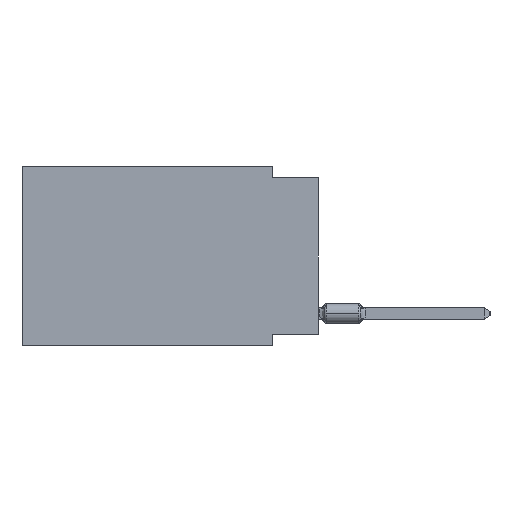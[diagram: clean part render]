
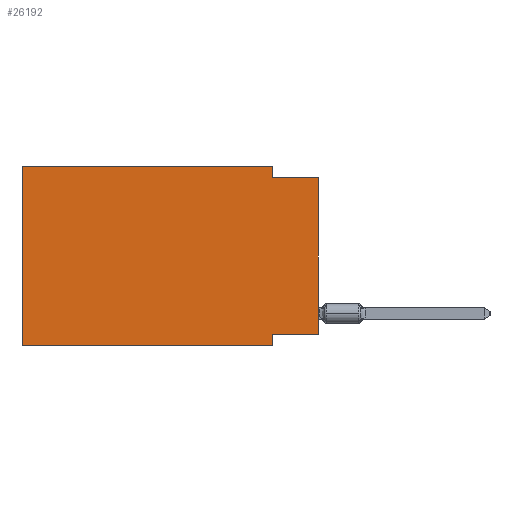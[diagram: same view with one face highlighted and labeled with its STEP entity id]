
A CAD part, left-side view. The second image highlights one B-rep face of the part: STEP entity #26192.
In plain terms, the highlighted planar face has unit normal (-1, 0, 0).
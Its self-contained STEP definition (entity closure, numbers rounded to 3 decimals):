
#17 = LINE ( 'NONE', #34394, #35979 ) ;
#1350 = EDGE_CURVE ( 'NONE', #41954, #53460, #18862, .T. ) ;
#2189 = LINE ( 'NONE', #27979, #35360 ) ;
#2396 = VERTEX_POINT ( 'NONE', #54322 ) ;
#2655 = AXIS2_PLACEMENT_3D ( 'NONE', #14996, #14698, #49918 ) ;
#2933 = CARTESIAN_POINT ( 'NONE',  ( 0., 0., -9.271 ) ) ;
#3360 = CARTESIAN_POINT ( 'NONE',  ( 0., 2.54, -9.906 ) ) ;
#4289 = CARTESIAN_POINT ( 'NONE',  ( 0., 2.54, 0. ) ) ;
#4582 = VECTOR ( 'NONE', #33559, 1000. ) ;
#6102 = PLANE ( 'NONE',  #2655 ) ;
#6469 = DIRECTION ( 'NONE',  ( 0., -1., 0. ) ) ;
#6684 = FACE_OUTER_BOUND ( 'NONE', #40012, .T. ) ;
#9177 = DIRECTION ( 'NONE',  ( 0., 0., 1. ) ) ;
#11233 = VECTOR ( 'NONE', #36967, 1000. ) ;
#11398 = DIRECTION ( 'NONE',  ( 0., 0., -1. ) ) ;
#14305 = ORIENTED_EDGE ( 'NONE', *, *, #56069, .F. ) ;
#14698 = DIRECTION ( 'NONE',  ( 1., 0., 0. ) ) ;
#14996 = CARTESIAN_POINT ( 'NONE',  ( 0., 16.383, 0. ) ) ;
#16462 = CARTESIAN_POINT ( 'NONE',  ( 0., 0., -0.635 ) ) ;
#17067 = ORIENTED_EDGE ( 'NONE', *, *, #1350, .T. ) ;
#17804 = ORIENTED_EDGE ( 'NONE', *, *, #56601, .F. ) ;
#18772 = ORIENTED_EDGE ( 'NONE', *, *, #55075, .F. ) ;
#18862 = LINE ( 'NONE', #40323, #44208 ) ;
#18875 = LINE ( 'NONE', #53771, #22609 ) ;
#19514 = LINE ( 'NONE', #46384, #11233 ) ;
#19991 = VERTEX_POINT ( 'NONE', #52858 ) ;
#20085 = EDGE_CURVE ( 'NONE', #2396, #51063, #2189, .T. ) ;
#20477 = CARTESIAN_POINT ( 'NONE',  ( 0., 0., -0.635 ) ) ;
#20501 = EDGE_CURVE ( 'NONE', #51063, #19991, #18875, .T. ) ;
#20952 = CARTESIAN_POINT ( 'NONE',  ( 0., 2.54, -9.906 ) ) ;
#22609 = VECTOR ( 'NONE', #27759, 1000. ) ;
#24961 = ORIENTED_EDGE ( 'NONE', *, *, #20501, .F. ) ;
#25992 = VERTEX_POINT ( 'NONE', #33649 ) ;
#26192 = ADVANCED_FACE ( 'NONE', ( #6684 ), #6102, .F. ) ;
#27759 = DIRECTION ( 'NONE',  ( 0., 0., -1. ) ) ;
#27979 = CARTESIAN_POINT ( 'NONE',  ( 0., 16.383, 0. ) ) ;
#29601 = CARTESIAN_POINT ( 'NONE',  ( 0., 2.54, -9.271 ) ) ;
#30923 = VERTEX_POINT ( 'NONE', #29601 ) ;
#33559 = DIRECTION ( 'NONE',  ( 0., 1., 0. ) ) ;
#33649 = CARTESIAN_POINT ( 'NONE',  ( 0., 16.383, -9.906 ) ) ;
#34031 = ORIENTED_EDGE ( 'NONE', *, *, #41405, .F. ) ;
#34394 = CARTESIAN_POINT ( 'NONE',  ( 0., 16.383, 0. ) ) ;
#35360 = VECTOR ( 'NONE', #6469, 1000. ) ;
#35979 = VECTOR ( 'NONE', #9177, 1000. ) ;
#36967 = DIRECTION ( 'NONE',  ( 0., -1., 0. ) ) ;
#40012 = EDGE_LOOP ( 'NONE', ( #17067, #17804, #24961, #41286, #34031, #43283, #14305, #18772 ) ) ;
#40323 = CARTESIAN_POINT ( 'NONE',  ( 0., 0., 0. ) ) ;
#41286 = ORIENTED_EDGE ( 'NONE', *, *, #20085, .F. ) ;
#41405 = EDGE_CURVE ( 'NONE', #25992, #2396, #17, .T. ) ;
#41954 = VERTEX_POINT ( 'NONE', #54560 ) ;
#42525 = LINE ( 'NONE', #16462, #52257 ) ;
#42582 = LINE ( 'NONE', #3360, #53116 ) ;
#43283 = ORIENTED_EDGE ( 'NONE', *, *, #50846, .T. ) ;
#44208 = VECTOR ( 'NONE', #44613, 1000. ) ;
#44613 = DIRECTION ( 'NONE',  ( 0., 0., 1. ) ) ;
#46384 = CARTESIAN_POINT ( 'NONE',  ( 0., 16.383, -9.906 ) ) ;
#46684 = VERTEX_POINT ( 'NONE', #20952 ) ;
#49918 = DIRECTION ( 'NONE',  ( 0., 0., -1. ) ) ;
#50846 = EDGE_CURVE ( 'NONE', #25992, #46684, #19514, .T. ) ;
#51063 = VERTEX_POINT ( 'NONE', #4289 ) ;
#52257 = VECTOR ( 'NONE', #56518, 1000. ) ;
#52858 = CARTESIAN_POINT ( 'NONE',  ( 0., 2.54, -0.635 ) ) ;
#53116 = VECTOR ( 'NONE', #11398, 1000. ) ;
#53460 = VERTEX_POINT ( 'NONE', #20477 ) ;
#53771 = CARTESIAN_POINT ( 'NONE',  ( 0., 2.54, 0. ) ) ;
#54322 = CARTESIAN_POINT ( 'NONE',  ( 0., 16.383, 0. ) ) ;
#54560 = CARTESIAN_POINT ( 'NONE',  ( 0., 0., -9.271 ) ) ;
#55075 = EDGE_CURVE ( 'NONE', #41954, #30923, #55886, .T. ) ;
#55886 = LINE ( 'NONE', #2933, #4582 ) ;
#56069 = EDGE_CURVE ( 'NONE', #30923, #46684, #42582, .T. ) ;
#56518 = DIRECTION ( 'NONE',  ( 0., -1., 0. ) ) ;
#56601 = EDGE_CURVE ( 'NONE', #19991, #53460, #42525, .T. ) ;
